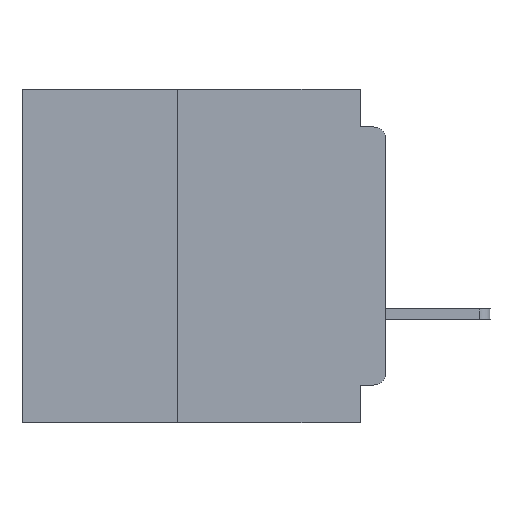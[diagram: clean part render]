
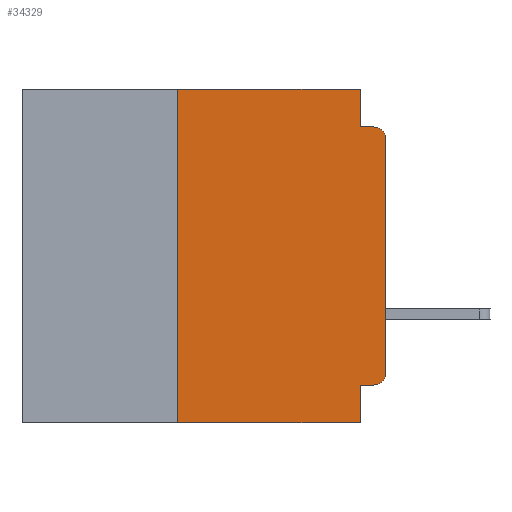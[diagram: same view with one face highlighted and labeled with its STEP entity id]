
A CAD part, left-side view. The second image highlights one B-rep face of the part: STEP entity #34329.
In plain terms, the highlighted planar face has unit normal (-1, 0, 0).
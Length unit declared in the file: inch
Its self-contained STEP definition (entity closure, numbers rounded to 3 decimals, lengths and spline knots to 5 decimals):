
#968 = CARTESIAN_POINT ( 'NONE',  ( 0., 0.015, -0.355 ) ) ;
#1062 = EDGE_CURVE ( 'NONE', #30746, #32575, #8785, .T. ) ;
#1235 = CARTESIAN_POINT ( 'NONE',  ( 0., 0.031, -0.4 ) ) ;
#1241 = VECTOR ( 'NONE', #32480, 39.37008 ) ;
#1901 = VERTEX_POINT ( 'NONE', #26807 ) ;
#2191 = ORIENTED_EDGE ( 'NONE', *, *, #57584, .F. ) ;
#2786 = VECTOR ( 'NONE', #29343, 39.37008 ) ;
#4205 = DIRECTION ( 'NONE',  ( 0., 0., 1. ) ) ;
#7302 = CARTESIAN_POINT ( 'NONE',  ( 0., 0.015, -0.34 ) ) ;
#8176 = VERTEX_POINT ( 'NONE', #19546 ) ;
#8785 = LINE ( 'NONE', #49528, #18214 ) ;
#10223 = LINE ( 'NONE', #1235, #33453 ) ;
#10795 = DIRECTION ( 'NONE',  ( 0., -1., 0. ) ) ;
#11956 = DIRECTION ( 'NONE',  ( 0., 0., -1. ) ) ;
#12195 = CARTESIAN_POINT ( 'NONE',  ( 0., 0.25, 0. ) ) ;
#12251 = ORIENTED_EDGE ( 'NONE', *, *, #37305, .T. ) ;
#12497 = CARTESIAN_POINT ( 'NONE',  ( 0., 0.437, 0. ) ) ;
#14117 = EDGE_CURVE ( 'NONE', #1901, #44373, #41047, .T. ) ;
#16352 = ORIENTED_EDGE ( 'NONE', *, *, #14117, .F. ) ;
#16403 = CARTESIAN_POINT ( 'NONE',  ( 0., 0.031, 0. ) ) ;
#16865 = CIRCLE ( 'NONE', #58155, 0.015 ) ;
#18214 = VECTOR ( 'NONE', #50550, 39.37008 ) ;
#19163 = AXIS2_PLACEMENT_3D ( 'NONE', #7302, #39578, #11956 ) ;
#19546 = CARTESIAN_POINT ( 'NONE',  ( 0., 0.031, -0.355 ) ) ;
#19649 = VERTEX_POINT ( 'NONE', #30952 ) ;
#19857 = ORIENTED_EDGE ( 'NONE', *, *, #38366, .F. ) ;
#20520 = ORIENTED_EDGE ( 'NONE', *, *, #50834, .F. ) ;
#20586 = VERTEX_POINT ( 'NONE', #33081 ) ;
#21402 = AXIS2_PLACEMENT_3D ( 'NONE', #12497, #58180, #31150 ) ;
#21930 = ORIENTED_EDGE ( 'NONE', *, *, #1062, .T. ) ;
#22203 = CARTESIAN_POINT ( 'NONE',  ( 0., 0.031, -0.045 ) ) ;
#22337 = VECTOR ( 'NONE', #32757, 39.37008 ) ;
#24263 = DIRECTION ( 'NONE',  ( -1., 0., 0. ) ) ;
#24693 = CARTESIAN_POINT ( 'NONE',  ( 0., 0., -0.355 ) ) ;
#25853 = ORIENTED_EDGE ( 'NONE', *, *, #50262, .T. ) ;
#26524 = PLANE ( 'NONE',  #21402 ) ;
#26807 = CARTESIAN_POINT ( 'NONE',  ( 0., 0.25, -0.4 ) ) ;
#27820 = CARTESIAN_POINT ( 'NONE',  ( 0., 0., -0.045 ) ) ;
#28079 = CARTESIAN_POINT ( 'NONE',  ( 0., 0.437, -0.4 ) ) ;
#28912 = VECTOR ( 'NONE', #4205, 39.37008 ) ;
#29343 = DIRECTION ( 'NONE',  ( 0., 1., 0. ) ) ;
#30119 = EDGE_LOOP ( 'NONE', ( #21930, #52006, #20520, #43217, #19857, #16352, #25853, #2191, #43173, #12251 ) ) ;
#30136 = CARTESIAN_POINT ( 'NONE',  ( 0., 0.031, -0.4 ) ) ;
#30746 = VERTEX_POINT ( 'NONE', #51750 ) ;
#30952 = CARTESIAN_POINT ( 'NONE',  ( 0., 0.031, 0. ) ) ;
#31150 = DIRECTION ( 'NONE',  ( 0., 0., -1. ) ) ;
#31978 = VECTOR ( 'NONE', #48378, 39.37008 ) ;
#32480 = DIRECTION ( 'NONE',  ( 0., -1., 0. ) ) ;
#32575 = VERTEX_POINT ( 'NONE', #51338 ) ;
#32757 = DIRECTION ( 'NONE',  ( 0., -1., 0. ) ) ;
#33081 = CARTESIAN_POINT ( 'NONE',  ( 0., 0.015, -0.045 ) ) ;
#33453 = VECTOR ( 'NONE', #56028, 39.37008 ) ;
#34329 = ADVANCED_FACE ( 'NONE', ( #35254 ), #26524, .F. ) ;
#34629 = VERTEX_POINT ( 'NONE', #968 ) ;
#34870 = CIRCLE ( 'NONE', #19163, 0.015 ) ;
#35254 = FACE_OUTER_BOUND ( 'NONE', #30119, .T. ) ;
#36343 = CARTESIAN_POINT ( 'NONE',  ( 0., 0.25, -0.4 ) ) ;
#37305 = EDGE_CURVE ( 'NONE', #34629, #30746, #34870, .T. ) ;
#38091 = LINE ( 'NONE', #27820, #1241 ) ;
#38170 = LINE ( 'NONE', #24693, #2786 ) ;
#38366 = EDGE_CURVE ( 'NONE', #44373, #19649, #51974, .T. ) ;
#39578 = DIRECTION ( 'NONE',  ( -1., 0., 0. ) ) ;
#40917 = VERTEX_POINT ( 'NONE', #30136 ) ;
#41047 = LINE ( 'NONE', #36343, #28912 ) ;
#42615 = LINE ( 'NONE', #16403, #31978 ) ;
#42786 = EDGE_CURVE ( 'NONE', #34629, #8176, #38170, .T. ) ;
#43000 = CARTESIAN_POINT ( 'NONE',  ( 0., 0.437, 0. ) ) ;
#43173 = ORIENTED_EDGE ( 'NONE', *, *, #42786, .F. ) ;
#43217 = ORIENTED_EDGE ( 'NONE', *, *, #46582, .F. ) ;
#44373 = VERTEX_POINT ( 'NONE', #12195 ) ;
#46582 = EDGE_CURVE ( 'NONE', #19649, #56635, #42615, .T. ) ;
#46585 = LINE ( 'NONE', #28079, #22337 ) ;
#48378 = DIRECTION ( 'NONE',  ( 0., 0., -1. ) ) ;
#49168 = VECTOR ( 'NONE', #10795, 39.37008 ) ;
#49528 = CARTESIAN_POINT ( 'NONE',  ( 0., 0., 0. ) ) ;
#50262 = EDGE_CURVE ( 'NONE', #1901, #40917, #46585, .T. ) ;
#50550 = DIRECTION ( 'NONE',  ( 0., 0., 1. ) ) ;
#50834 = EDGE_CURVE ( 'NONE', #56635, #20586, #38091, .T. ) ;
#51338 = CARTESIAN_POINT ( 'NONE',  ( 0., 0., -0.06 ) ) ;
#51427 = CARTESIAN_POINT ( 'NONE',  ( 0., 0.015, -0.06 ) ) ;
#51750 = CARTESIAN_POINT ( 'NONE',  ( 0., 0., -0.34 ) ) ;
#51974 = LINE ( 'NONE', #43000, #49168 ) ;
#52006 = ORIENTED_EDGE ( 'NONE', *, *, #53045, .T. ) ;
#53045 = EDGE_CURVE ( 'NONE', #32575, #20586, #16865, .T. ) ;
#55956 = DIRECTION ( 'NONE',  ( 0., 0., -1. ) ) ;
#56028 = DIRECTION ( 'NONE',  ( 0., 0., -1. ) ) ;
#56635 = VERTEX_POINT ( 'NONE', #22203 ) ;
#57584 = EDGE_CURVE ( 'NONE', #8176, #40917, #10223, .T. ) ;
#58155 = AXIS2_PLACEMENT_3D ( 'NONE', #51427, #24263, #55956 ) ;
#58180 = DIRECTION ( 'NONE',  ( 1., 0., 0. ) ) ;
